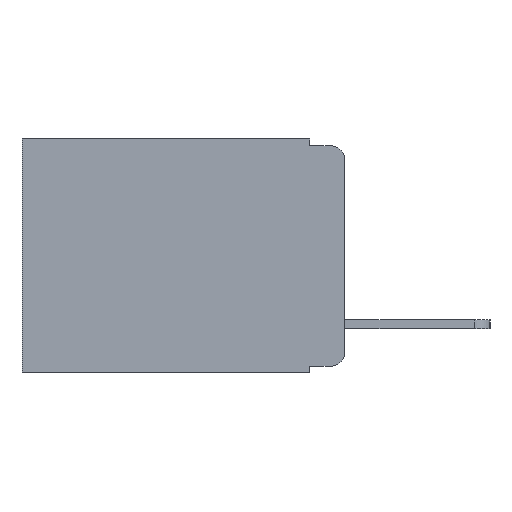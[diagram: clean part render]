
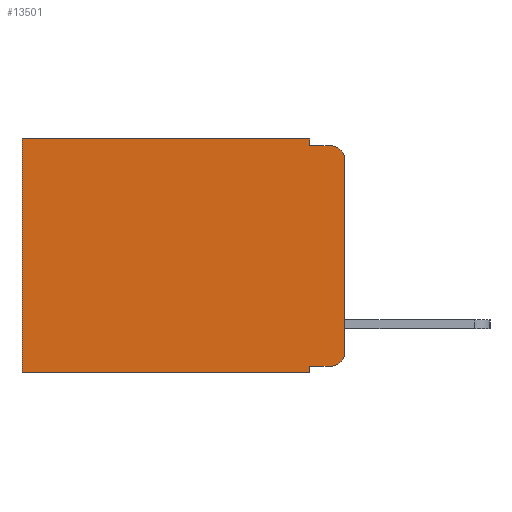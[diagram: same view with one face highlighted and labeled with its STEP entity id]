
A CAD part, left-side view. The second image highlights one B-rep face of the part: STEP entity #13501.
In plain terms, the highlighted planar face has unit normal (-1, 0, 0).
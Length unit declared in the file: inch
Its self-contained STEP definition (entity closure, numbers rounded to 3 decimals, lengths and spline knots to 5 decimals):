
#13 = DIRECTION ( 'NONE',  ( 0., 0., -1. ) ) ;
#135 = ORIENTED_EDGE ( 'NONE', *, *, #10345, .F. ) ;
#1065 = CARTESIAN_POINT ( 'NONE',  ( 0.298, 0.02, -0.01 ) ) ;
#1469 = CARTESIAN_POINT ( 'NONE',  ( 0.298, 0.051, -0.333 ) ) ;
#1589 = LINE ( 'NONE', #18112, #10265 ) ;
#2045 = AXIS2_PLACEMENT_3D ( 'NONE', #10646, #12159, #2585 ) ;
#2424 = VERTEX_POINT ( 'NONE', #9000 ) ;
#2571 = VECTOR ( 'NONE', #12237, 39.37008 ) ;
#2585 = DIRECTION ( 'NONE',  ( 0., 0., -1. ) ) ;
#2729 = EDGE_CURVE ( 'NONE', #2424, #11518, #4615, .T. ) ;
#2757 = ORIENTED_EDGE ( 'NONE', *, *, #9319, .F. ) ;
#2785 = ORIENTED_EDGE ( 'NONE', *, *, #14713, .T. ) ;
#3023 = CARTESIAN_POINT ( 'NONE',  ( 0.298, 0., -0.03 ) ) ;
#3394 = LINE ( 'NONE', #18255, #15129 ) ;
#3515 = EDGE_LOOP ( 'NONE', ( #3813, #4022, #135, #2757, #2785, #8282, #8068, #8243, #8929, #8033 ) ) ;
#3728 = CARTESIAN_POINT ( 'NONE',  ( 0.298, 0.051, -0.343 ) ) ;
#3813 = ORIENTED_EDGE ( 'NONE', *, *, #13440, .F. ) ;
#4022 = ORIENTED_EDGE ( 'NONE', *, *, #11396, .T. ) ;
#4243 = CARTESIAN_POINT ( 'NONE',  ( 0.298, 0., -0.343 ) ) ;
#4615 = CIRCLE ( 'NONE', #20061, 0.02 ) ;
#4837 = CARTESIAN_POINT ( 'NONE',  ( 0.298, 0.473, -0.343 ) ) ;
#4969 = EDGE_CURVE ( 'NONE', #12047, #2424, #8499, .T. ) ;
#5211 = DIRECTION ( 'NONE',  ( 0., 0., -1. ) ) ;
#5664 = FACE_OUTER_BOUND ( 'NONE', #3515, .T. ) ;
#6035 = EDGE_CURVE ( 'NONE', #12047, #12475, #20310, .T. ) ;
#6055 = VECTOR ( 'NONE', #6272, 39.37008 ) ;
#6072 = LINE ( 'NONE', #14569, #18674 ) ;
#6272 = DIRECTION ( 'NONE',  ( 0., -1., 0. ) ) ;
#6385 = VERTEX_POINT ( 'NONE', #17467 ) ;
#7122 = EDGE_CURVE ( 'NONE', #17059, #16251, #1589, .T. ) ;
#7365 = DIRECTION ( 'NONE',  ( 0., 1., 0. ) ) ;
#7896 = VERTEX_POINT ( 'NONE', #13883 ) ;
#8033 = ORIENTED_EDGE ( 'NONE', *, *, #2729, .T. ) ;
#8068 = ORIENTED_EDGE ( 'NONE', *, *, #20034, .F. ) ;
#8243 = ORIENTED_EDGE ( 'NONE', *, *, #6035, .F. ) ;
#8282 = ORIENTED_EDGE ( 'NONE', *, *, #7122, .T. ) ;
#8412 = CARTESIAN_POINT ( 'NONE',  ( 0.298, 0.473, 0. ) ) ;
#8499 = LINE ( 'NONE', #1469, #12125 ) ;
#8929 = ORIENTED_EDGE ( 'NONE', *, *, #4969, .T. ) ;
#9000 = CARTESIAN_POINT ( 'NONE',  ( 0.298, 0.02, -0.333 ) ) ;
#9319 = EDGE_CURVE ( 'NONE', #7896, #6385, #6072, .T. ) ;
#9579 = CIRCLE ( 'NONE', #15606, 0.02 ) ;
#9899 = VECTOR ( 'NONE', #7365, 39.37008 ) ;
#9980 = DIRECTION ( 'NONE',  ( -1., 0., 0. ) ) ;
#10002 = CARTESIAN_POINT ( 'NONE',  ( 0.298, 0.051, 0. ) ) ;
#10265 = VECTOR ( 'NONE', #10287, 39.37008 ) ;
#10287 = DIRECTION ( 'NONE',  ( 0., 0., -1. ) ) ;
#10333 = LINE ( 'NONE', #18842, #6055 ) ;
#10345 = EDGE_CURVE ( 'NONE', #6385, #13066, #10333, .T. ) ;
#10646 = CARTESIAN_POINT ( 'NONE',  ( 0.298, 0., 0. ) ) ;
#11122 = VERTEX_POINT ( 'NONE', #3023 ) ;
#11158 = LINE ( 'NONE', #4243, #2571 ) ;
#11396 = EDGE_CURVE ( 'NONE', #11122, #13066, #9579, .T. ) ;
#11406 = DIRECTION ( 'NONE',  ( 0., 0., -1. ) ) ;
#11518 = VERTEX_POINT ( 'NONE', #17931 ) ;
#11644 = DIRECTION ( 'NONE',  ( -1., 0., 0. ) ) ;
#11688 = CARTESIAN_POINT ( 'NONE',  ( 0.298, 0.02, -0.313 ) ) ;
#11925 = DIRECTION ( 'NONE',  ( 0., 0., -1. ) ) ;
#11969 = VECTOR ( 'NONE', #5211, 39.37008 ) ;
#12047 = VERTEX_POINT ( 'NONE', #14273 ) ;
#12125 = VECTOR ( 'NONE', #12774, 39.37008 ) ;
#12159 = DIRECTION ( 'NONE',  ( 1., 0., 0. ) ) ;
#12237 = DIRECTION ( 'NONE',  ( 0., 1., 0. ) ) ;
#12475 = VERTEX_POINT ( 'NONE', #3728 ) ;
#12774 = DIRECTION ( 'NONE',  ( 0., -1., 0. ) ) ;
#13066 = VERTEX_POINT ( 'NONE', #1065 ) ;
#13440 = EDGE_CURVE ( 'NONE', #11122, #11518, #3394, .T. ) ;
#13501 = ADVANCED_FACE ( 'NONE', ( #5664 ), #16918, .F. ) ;
#13883 = CARTESIAN_POINT ( 'NONE',  ( 0.298, 0.051, 0. ) ) ;
#14273 = CARTESIAN_POINT ( 'NONE',  ( 0.298, 0.051, -0.333 ) ) ;
#14569 = CARTESIAN_POINT ( 'NONE',  ( 0.298, 0.051, 0. ) ) ;
#14713 = EDGE_CURVE ( 'NONE', #7896, #17059, #18230, .T. ) ;
#15129 = VECTOR ( 'NONE', #19799, 39.37008 ) ;
#15606 = AXIS2_PLACEMENT_3D ( 'NONE', #19337, #9980, #13 ) ;
#16251 = VERTEX_POINT ( 'NONE', #4837 ) ;
#16870 = CARTESIAN_POINT ( 'NONE',  ( 0.298, 0., 0. ) ) ;
#16918 = PLANE ( 'NONE',  #2045 ) ;
#17059 = VERTEX_POINT ( 'NONE', #8412 ) ;
#17467 = CARTESIAN_POINT ( 'NONE',  ( 0.298, 0.051, -0.01 ) ) ;
#17931 = CARTESIAN_POINT ( 'NONE',  ( 0.298, 0., -0.313 ) ) ;
#18112 = CARTESIAN_POINT ( 'NONE',  ( 0.298, 0.473, 0. ) ) ;
#18230 = LINE ( 'NONE', #16870, #9899 ) ;
#18255 = CARTESIAN_POINT ( 'NONE',  ( 0.298, 0., 0. ) ) ;
#18674 = VECTOR ( 'NONE', #11406, 39.37008 ) ;
#18842 = CARTESIAN_POINT ( 'NONE',  ( 0.298, 0.051, -0.01 ) ) ;
#19337 = CARTESIAN_POINT ( 'NONE',  ( 0.298, 0.02, -0.03 ) ) ;
#19799 = DIRECTION ( 'NONE',  ( 0., 0., -1. ) ) ;
#20034 = EDGE_CURVE ( 'NONE', #12475, #16251, #11158, .T. ) ;
#20061 = AXIS2_PLACEMENT_3D ( 'NONE', #11688, #11644, #11925 ) ;
#20310 = LINE ( 'NONE', #10002, #11969 ) ;
